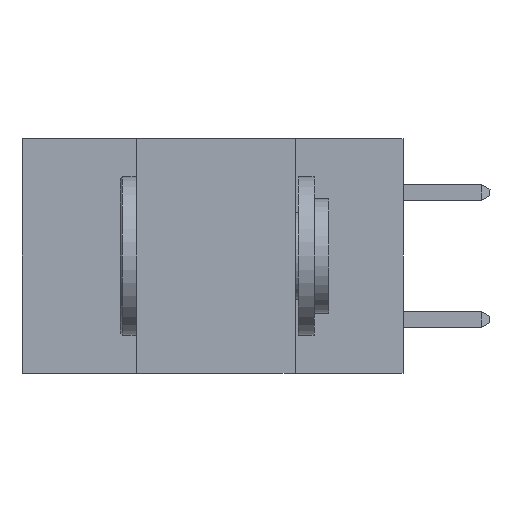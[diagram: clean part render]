
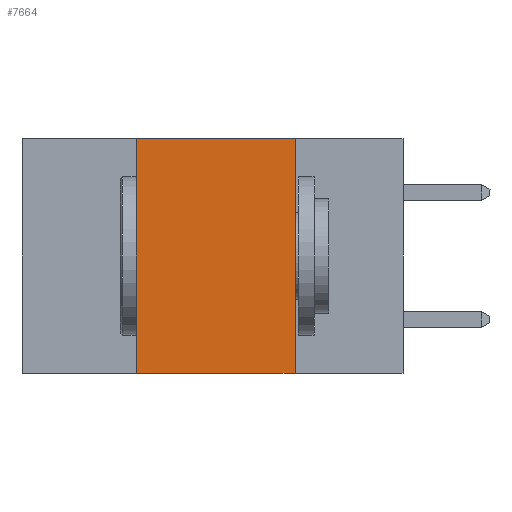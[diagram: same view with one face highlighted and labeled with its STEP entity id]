
A CAD part, left-side view. The second image highlights one B-rep face of the part: STEP entity #7664.
In plain terms, the highlighted planar face has unit normal (-1, 0, 0).
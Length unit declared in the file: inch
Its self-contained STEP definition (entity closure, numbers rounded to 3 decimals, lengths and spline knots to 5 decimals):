
#600 = CARTESIAN_POINT ( 'NONE',  ( 0., 0.42, 0. ) ) ;
#692 = ORIENTED_EDGE ( 'NONE', *, *, #4521, .F. ) ;
#849 = EDGE_CURVE ( 'NONE', #3938, #5766, #3987, .T. ) ;
#1187 = VERTEX_POINT ( 'NONE', #600 ) ;
#1257 = LINE ( 'NONE', #2657, #8977 ) ;
#2057 = VECTOR ( 'NONE', #4089, 39.37008 ) ;
#2355 = PLANE ( 'NONE',  #5193 ) ;
#2454 = CARTESIAN_POINT ( 'NONE',  ( 0., 0.42, -0.37 ) ) ;
#2620 = DIRECTION ( 'NONE',  ( 0., -1., 0. ) ) ;
#2657 = CARTESIAN_POINT ( 'NONE',  ( 0., 0.6, 0. ) ) ;
#2700 = VECTOR ( 'NONE', #8584, 39.37008 ) ;
#3039 = ORIENTED_EDGE ( 'NONE', *, *, #8357, .F. ) ;
#3739 = EDGE_LOOP ( 'NONE', ( #7910, #692, #3039, #7181 ) ) ;
#3839 = VERTEX_POINT ( 'NONE', #9440 ) ;
#3938 = VERTEX_POINT ( 'NONE', #2454 ) ;
#3987 = LINE ( 'NONE', #8228, #2057 ) ;
#4002 = CARTESIAN_POINT ( 'NONE',  ( 0., 0.6, 0. ) ) ;
#4050 = DIRECTION ( 'NONE',  ( 0., 0., -1. ) ) ;
#4063 = VECTOR ( 'NONE', #4050, 39.37008 ) ;
#4089 = DIRECTION ( 'NONE',  ( 0., -1., 0. ) ) ;
#4213 = CARTESIAN_POINT ( 'NONE',  ( 0., 0.17, 0. ) ) ;
#4437 = CARTESIAN_POINT ( 'NONE',  ( 0., 0.42, 0. ) ) ;
#4457 = EDGE_CURVE ( 'NONE', #3839, #5766, #8096, .T. ) ;
#4521 = EDGE_CURVE ( 'NONE', #1187, #3839, #1257, .T. ) ;
#4873 = DIRECTION ( 'NONE',  ( 0., 0., -1. ) ) ;
#4926 = LINE ( 'NONE', #4437, #2700 ) ;
#5193 = AXIS2_PLACEMENT_3D ( 'NONE', #4002, #8910, #4873 ) ;
#5766 = VERTEX_POINT ( 'NONE', #8372 ) ;
#7181 = ORIENTED_EDGE ( 'NONE', *, *, #849, .T. ) ;
#7664 = ADVANCED_FACE ( 'NONE', ( #9592 ), #2355, .F. ) ;
#7910 = ORIENTED_EDGE ( 'NONE', *, *, #4457, .F. ) ;
#8096 = LINE ( 'NONE', #4213, #4063 ) ;
#8228 = CARTESIAN_POINT ( 'NONE',  ( 0., 0.6, -0.37 ) ) ;
#8357 = EDGE_CURVE ( 'NONE', #3938, #1187, #4926, .T. ) ;
#8372 = CARTESIAN_POINT ( 'NONE',  ( 0., 0.17, -0.37 ) ) ;
#8584 = DIRECTION ( 'NONE',  ( 0., 0., 1. ) ) ;
#8910 = DIRECTION ( 'NONE',  ( 1., 0., 0. ) ) ;
#8977 = VECTOR ( 'NONE', #2620, 39.37008 ) ;
#9440 = CARTESIAN_POINT ( 'NONE',  ( 0., 0.17, 0. ) ) ;
#9592 = FACE_OUTER_BOUND ( 'NONE', #3739, .T. ) ;
